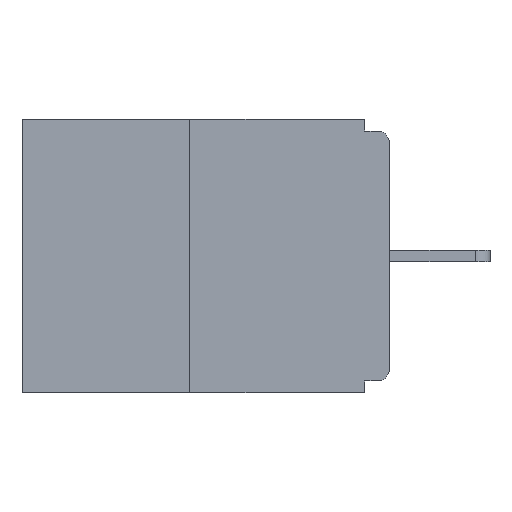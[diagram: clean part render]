
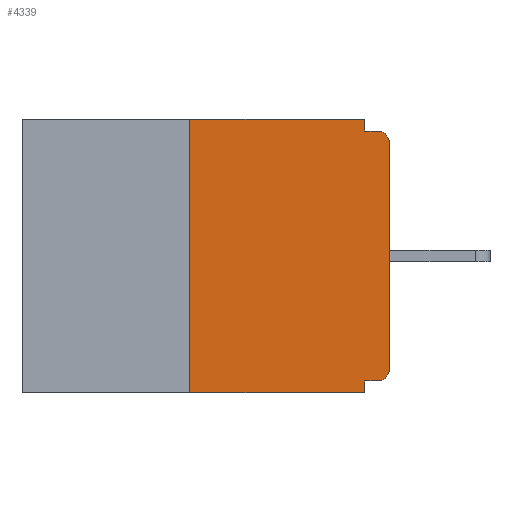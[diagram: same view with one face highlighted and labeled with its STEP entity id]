
A CAD part, left-side view. The second image highlights one B-rep face of the part: STEP entity #4339.
In plain terms, the highlighted planar face has unit normal (-1, 0, 0).
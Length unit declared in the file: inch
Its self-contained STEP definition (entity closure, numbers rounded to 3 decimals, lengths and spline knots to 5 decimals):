
#27 = VERTEX_POINT ( 'NONE', #15493 ) ;
#94 = VERTEX_POINT ( 'NONE', #8859 ) ;
#173 = DIRECTION ( 'NONE',  ( 0., 0., -1. ) ) ;
#178 = AXIS2_PLACEMENT_3D ( 'NONE', #13683, #3943, #4197 ) ;
#625 = VERTEX_POINT ( 'NONE', #8425 ) ;
#916 = CARTESIAN_POINT ( 'NONE',  ( 0., 0.46, -0.343 ) ) ;
#1174 = DIRECTION ( 'NONE',  ( 0., 0., 1. ) ) ;
#1537 = CARTESIAN_POINT ( 'NONE',  ( 0., 0.25, 0. ) ) ;
#1797 = LINE ( 'NONE', #916, #11087 ) ;
#2031 = EDGE_CURVE ( 'NONE', #8666, #3185, #6723, .T. ) ;
#2107 = EDGE_CURVE ( 'NONE', #12139, #94, #5539, .T. ) ;
#2795 = DIRECTION ( 'NONE',  ( 0., 0., -1. ) ) ;
#3122 = EDGE_CURVE ( 'NONE', #11442, #27, #10634, .T. ) ;
#3185 = VERTEX_POINT ( 'NONE', #15031 ) ;
#3393 = VECTOR ( 'NONE', #2795, 39.37008 ) ;
#3517 = LINE ( 'NONE', #6525, #6478 ) ;
#3921 = VECTOR ( 'NONE', #1174, 39.37008 ) ;
#3943 = DIRECTION ( 'NONE',  ( -1., 0., 0. ) ) ;
#3975 = AXIS2_PLACEMENT_3D ( 'NONE', #9318, #9849, #9819 ) ;
#4117 = DIRECTION ( 'NONE',  ( 0., -1., 0. ) ) ;
#4197 = DIRECTION ( 'NONE',  ( 0., 0., -1. ) ) ;
#4339 = ADVANCED_FACE ( 'NONE', ( #15057 ), #9373, .F. ) ;
#4640 = CARTESIAN_POINT ( 'NONE',  ( 0., 0.015, -0.328 ) ) ;
#5469 = ORIENTED_EDGE ( 'NONE', *, *, #13038, .F. ) ;
#5508 = VERTEX_POINT ( 'NONE', #7858 ) ;
#5539 = CIRCLE ( 'NONE', #178, 0.015 ) ;
#5787 = CIRCLE ( 'NONE', #10942, 0.015 ) ;
#6186 = CARTESIAN_POINT ( 'NONE',  ( 0., 0., 0. ) ) ;
#6478 = VECTOR ( 'NONE', #7850, 39.37008 ) ;
#6525 = CARTESIAN_POINT ( 'NONE',  ( 0., 0.46, 0. ) ) ;
#6723 = LINE ( 'NONE', #15952, #9730 ) ;
#6784 = CARTESIAN_POINT ( 'NONE',  ( 0., 0., -0.328 ) ) ;
#7162 = ORIENTED_EDGE ( 'NONE', *, *, #14913, .F. ) ;
#7345 = ORIENTED_EDGE ( 'NONE', *, *, #2031, .F. ) ;
#7445 = ORIENTED_EDGE ( 'NONE', *, *, #14586, .T. ) ;
#7489 = DIRECTION ( 'NONE',  ( 0., 0., 1. ) ) ;
#7850 = DIRECTION ( 'NONE',  ( 0., -1., 0. ) ) ;
#7858 = CARTESIAN_POINT ( 'NONE',  ( 0., 0.031, -0.328 ) ) ;
#7865 = DIRECTION ( 'NONE',  ( -1., 0., 0. ) ) ;
#7897 = VERTEX_POINT ( 'NONE', #15549 ) ;
#8174 = EDGE_LOOP ( 'NONE', ( #12996, #14778, #9021, #5469, #7162, #12278, #7445, #8179, #10572, #7345 ) ) ;
#8179 = ORIENTED_EDGE ( 'NONE', *, *, #11821, .T. ) ;
#8378 = LINE ( 'NONE', #6186, #14579 ) ;
#8425 = CARTESIAN_POINT ( 'NONE',  ( 0., 0., -0.03 ) ) ;
#8666 = VERTEX_POINT ( 'NONE', #9627 ) ;
#8859 = CARTESIAN_POINT ( 'NONE',  ( 0., 0., -0.313 ) ) ;
#9005 = EDGE_CURVE ( 'NONE', #27, #8666, #3517, .T. ) ;
#9021 = ORIENTED_EDGE ( 'NONE', *, *, #12725, .T. ) ;
#9318 = CARTESIAN_POINT ( 'NONE',  ( 0., 0.46, 0. ) ) ;
#9373 = PLANE ( 'NONE',  #3975 ) ;
#9426 = VERTEX_POINT ( 'NONE', #10973 ) ;
#9558 = VECTOR ( 'NONE', #10642, 39.37008 ) ;
#9627 = CARTESIAN_POINT ( 'NONE',  ( 0., 0.031, 0. ) ) ;
#9730 = VECTOR ( 'NONE', #12655, 39.37008 ) ;
#9819 = DIRECTION ( 'NONE',  ( 0., 0., -1. ) ) ;
#9849 = DIRECTION ( 'NONE',  ( 1., 0., 0. ) ) ;
#9863 = DIRECTION ( 'NONE',  ( 0., -1., 0. ) ) ;
#10013 = EDGE_CURVE ( 'NONE', #3185, #9426, #15420, .T. ) ;
#10572 = ORIENTED_EDGE ( 'NONE', *, *, #10013, .F. ) ;
#10634 = LINE ( 'NONE', #1537, #3921 ) ;
#10642 = DIRECTION ( 'NONE',  ( 0., 1., 0. ) ) ;
#10942 = AXIS2_PLACEMENT_3D ( 'NONE', #15280, #7865, #173 ) ;
#10973 = CARTESIAN_POINT ( 'NONE',  ( 0., 0.015, -0.015 ) ) ;
#11087 = VECTOR ( 'NONE', #9863, 39.37008 ) ;
#11442 = VERTEX_POINT ( 'NONE', #14637 ) ;
#11821 = EDGE_CURVE ( 'NONE', #625, #9426, #5787, .T. ) ;
#12139 = VERTEX_POINT ( 'NONE', #4640 ) ;
#12278 = ORIENTED_EDGE ( 'NONE', *, *, #2107, .T. ) ;
#12655 = DIRECTION ( 'NONE',  ( 0., 0., -1. ) ) ;
#12725 = EDGE_CURVE ( 'NONE', #11442, #7897, #1797, .T. ) ;
#12832 = CARTESIAN_POINT ( 'NONE',  ( 0., 0.031, -0.343 ) ) ;
#12843 = LINE ( 'NONE', #6784, #9558 ) ;
#12996 = ORIENTED_EDGE ( 'NONE', *, *, #9005, .F. ) ;
#13038 = EDGE_CURVE ( 'NONE', #5508, #7897, #13439, .T. ) ;
#13439 = LINE ( 'NONE', #12832, #3393 ) ;
#13683 = CARTESIAN_POINT ( 'NONE',  ( 0., 0.015, -0.313 ) ) ;
#14579 = VECTOR ( 'NONE', #7489, 39.37008 ) ;
#14586 = EDGE_CURVE ( 'NONE', #94, #625, #8378, .T. ) ;
#14637 = CARTESIAN_POINT ( 'NONE',  ( 0., 0.25, -0.343 ) ) ;
#14778 = ORIENTED_EDGE ( 'NONE', *, *, #3122, .F. ) ;
#14913 = EDGE_CURVE ( 'NONE', #12139, #5508, #12843, .T. ) ;
#15031 = CARTESIAN_POINT ( 'NONE',  ( 0., 0.031, -0.015 ) ) ;
#15057 = FACE_OUTER_BOUND ( 'NONE', #8174, .T. ) ;
#15280 = CARTESIAN_POINT ( 'NONE',  ( 0., 0.015, -0.03 ) ) ;
#15420 = LINE ( 'NONE', #15432, #15779 ) ;
#15432 = CARTESIAN_POINT ( 'NONE',  ( 0., 0., -0.015 ) ) ;
#15493 = CARTESIAN_POINT ( 'NONE',  ( 0., 0.25, 0. ) ) ;
#15549 = CARTESIAN_POINT ( 'NONE',  ( 0., 0.031, -0.343 ) ) ;
#15779 = VECTOR ( 'NONE', #4117, 39.37008 ) ;
#15952 = CARTESIAN_POINT ( 'NONE',  ( 0., 0.031, 0. ) ) ;
